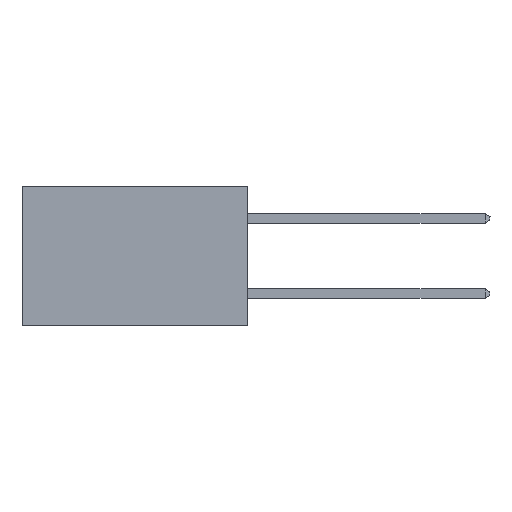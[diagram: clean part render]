
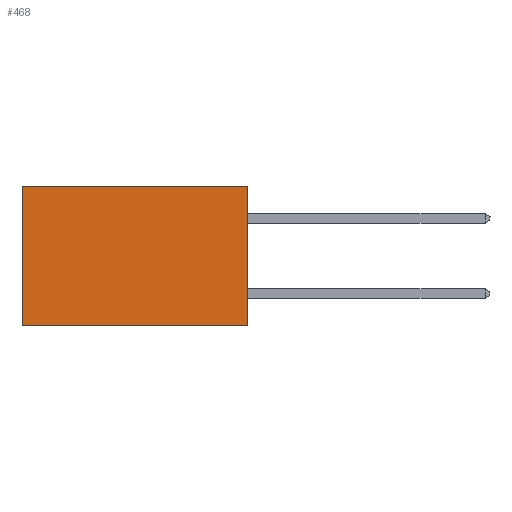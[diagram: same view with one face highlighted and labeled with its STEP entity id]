
A CAD part, left-side view. The second image highlights one B-rep face of the part: STEP entity #468.
In plain terms, the highlighted planar face has unit normal (-1, 0, 0).
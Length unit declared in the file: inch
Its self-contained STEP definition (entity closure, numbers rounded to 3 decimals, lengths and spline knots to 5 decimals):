
#188 = ORIENTED_EDGE ( 'NONE', *, *, #10133, .F. ) ;
#468 = ADVANCED_FACE ( 'NONE', ( #12120 ), #8830, .F. ) ;
#633 = DIRECTION ( 'NONE',  ( 0., 0., -1. ) ) ;
#742 = ORIENTED_EDGE ( 'NONE', *, *, #14669, .T. ) ;
#1202 = VECTOR ( 'NONE', #3025, 39.37008 ) ;
#1799 = LINE ( 'NONE', #10616, #1202 ) ;
#2371 = LINE ( 'NONE', #23673, #16979 ) ;
#3025 = DIRECTION ( 'NONE',  ( 0., 1., 0. ) ) ;
#3330 = VERTEX_POINT ( 'NONE', #15330 ) ;
#3446 = VECTOR ( 'NONE', #9909, 39.37008 ) ;
#6794 = LINE ( 'NONE', #24071, #21271 ) ;
#7194 = CARTESIAN_POINT ( 'NONE',  ( 0.298, 0., 0. ) ) ;
#7714 = ORIENTED_EDGE ( 'NONE', *, *, #18449, .F. ) ;
#8652 = EDGE_CURVE ( 'NONE', #8945, #16392, #2371, .T. ) ;
#8830 = PLANE ( 'NONE',  #15484 ) ;
#8945 = VERTEX_POINT ( 'NONE', #14195 ) ;
#8980 = DIRECTION ( 'NONE',  ( 0., 0., -1. ) ) ;
#9909 = DIRECTION ( 'NONE',  ( 0., 0., -1. ) ) ;
#10133 = EDGE_CURVE ( 'NONE', #8945, #3330, #22981, .T. ) ;
#10616 = CARTESIAN_POINT ( 'NONE',  ( 0.298, 0., -0.37 ) ) ;
#12120 = FACE_OUTER_BOUND ( 'NONE', #18801, .T. ) ;
#13447 = ORIENTED_EDGE ( 'NONE', *, *, #8652, .T. ) ;
#14195 = CARTESIAN_POINT ( 'NONE',  ( 0.298, 0., 0. ) ) ;
#14669 = EDGE_CURVE ( 'NONE', #16392, #16830, #6794, .T. ) ;
#15330 = CARTESIAN_POINT ( 'NONE',  ( 0.298, 0., -0.37 ) ) ;
#15484 = AXIS2_PLACEMENT_3D ( 'NONE', #7194, #15906, #633 ) ;
#15906 = DIRECTION ( 'NONE',  ( 1., 0., 0. ) ) ;
#16034 = DIRECTION ( 'NONE',  ( 0., 1., 0. ) ) ;
#16392 = VERTEX_POINT ( 'NONE', #21173 ) ;
#16830 = VERTEX_POINT ( 'NONE', #16923 ) ;
#16923 = CARTESIAN_POINT ( 'NONE',  ( 0.298, 0.6, -0.37 ) ) ;
#16979 = VECTOR ( 'NONE', #16034, 39.37008 ) ;
#18449 = EDGE_CURVE ( 'NONE', #3330, #16830, #1799, .T. ) ;
#18801 = EDGE_LOOP ( 'NONE', ( #742, #7714, #188, #13447 ) ) ;
#21173 = CARTESIAN_POINT ( 'NONE',  ( 0.298, 0.6, 0. ) ) ;
#21271 = VECTOR ( 'NONE', #8980, 39.37008 ) ;
#21948 = CARTESIAN_POINT ( 'NONE',  ( 0.298, 0., 0. ) ) ;
#22981 = LINE ( 'NONE', #21948, #3446 ) ;
#23673 = CARTESIAN_POINT ( 'NONE',  ( 0.298, 0., 0. ) ) ;
#24071 = CARTESIAN_POINT ( 'NONE',  ( 0.298, 0.6, 0. ) ) ;
